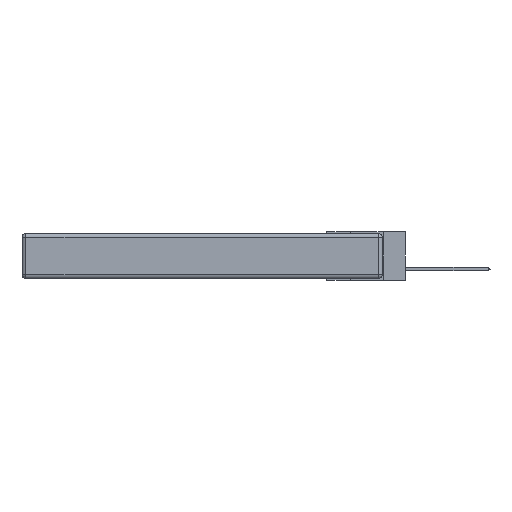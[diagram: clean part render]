
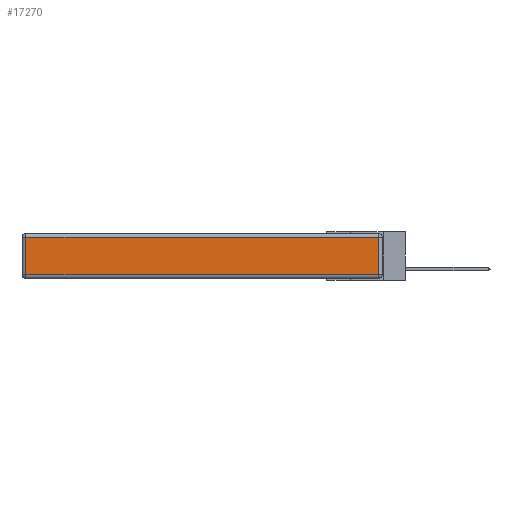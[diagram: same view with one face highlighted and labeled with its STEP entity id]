
A CAD part, left-side view. The second image highlights one B-rep face of the part: STEP entity #17270.
In plain terms, the highlighted planar face has unit normal (-1, 0, 0).
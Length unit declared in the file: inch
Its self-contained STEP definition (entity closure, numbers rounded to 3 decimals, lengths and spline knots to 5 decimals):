
#1890 = DIRECTION ( 'NONE',  ( 0., 0., -1. ) ) ;
#2254 = LINE ( 'NONE', #18075, #13479 ) ;
#3679 = DIRECTION ( 'NONE',  ( 0., -1., 0. ) ) ;
#4051 = LINE ( 'NONE', #5305, #10048 ) ;
#5305 = CARTESIAN_POINT ( 'NONE',  ( 0., 2.75, -0.03 ) ) ;
#6895 = VECTOR ( 'NONE', #1890, 39.37008 ) ;
#7994 = CARTESIAN_POINT ( 'NONE',  ( 0., 0., -0.343 ) ) ;
#8302 = EDGE_CURVE ( 'NONE', #24025, #23585, #4051, .T. ) ;
#10048 = VECTOR ( 'NONE', #16971, 39.37008 ) ;
#11535 = CARTESIAN_POINT ( 'NONE',  ( 0., 2.72, -0.313 ) ) ;
#12729 = EDGE_CURVE ( 'NONE', #23585, #23739, #26025, .T. ) ;
#13408 = CARTESIAN_POINT ( 'NONE',  ( 0., 2.72, -0.03 ) ) ;
#13479 = VECTOR ( 'NONE', #15864, 39.37008 ) ;
#14638 = EDGE_CURVE ( 'NONE', #25434, #24025, #2254, .T. ) ;
#15864 = DIRECTION ( 'NONE',  ( 0., 0., 1. ) ) ;
#16971 = DIRECTION ( 'NONE',  ( 0., 1., 0. ) ) ;
#17256 = DIRECTION ( 'NONE',  ( -1., 0., 0. ) ) ;
#17270 = ADVANCED_FACE ( 'NONE', ( #20361 ), #17362, .T. ) ;
#17362 = PLANE ( 'NONE',  #27589 ) ;
#18075 = CARTESIAN_POINT ( 'NONE',  ( 0., 0.03, -0.343 ) ) ;
#19526 = EDGE_CURVE ( 'NONE', #23739, #25434, #29280, .T. ) ;
#19808 = VECTOR ( 'NONE', #3679, 39.37008 ) ;
#20361 = FACE_OUTER_BOUND ( 'NONE', #20872, .T. ) ;
#20722 = CARTESIAN_POINT ( 'NONE',  ( 0., 2.72, -0.343 ) ) ;
#20872 = EDGE_LOOP ( 'NONE', ( #30886, #24087, #23037, #30581 ) ) ;
#22336 = CARTESIAN_POINT ( 'NONE',  ( 0., 0.03, -0.313 ) ) ;
#23037 = ORIENTED_EDGE ( 'NONE', *, *, #8302, .T. ) ;
#23585 = VERTEX_POINT ( 'NONE', #13408 ) ;
#23739 = VERTEX_POINT ( 'NONE', #11535 ) ;
#24025 = VERTEX_POINT ( 'NONE', #27990 ) ;
#24087 = ORIENTED_EDGE ( 'NONE', *, *, #14638, .T. ) ;
#24465 = CARTESIAN_POINT ( 'NONE',  ( 0., 0., -0.313 ) ) ;
#25434 = VERTEX_POINT ( 'NONE', #22336 ) ;
#26025 = LINE ( 'NONE', #20722, #6895 ) ;
#27589 = AXIS2_PLACEMENT_3D ( 'NONE', #7994, #17256, #29154 ) ;
#27990 = CARTESIAN_POINT ( 'NONE',  ( 0., 0.03, -0.03 ) ) ;
#29154 = DIRECTION ( 'NONE',  ( 0., 0., 1. ) ) ;
#29280 = LINE ( 'NONE', #24465, #19808 ) ;
#30581 = ORIENTED_EDGE ( 'NONE', *, *, #12729, .T. ) ;
#30886 = ORIENTED_EDGE ( 'NONE', *, *, #19526, .T. ) ;
